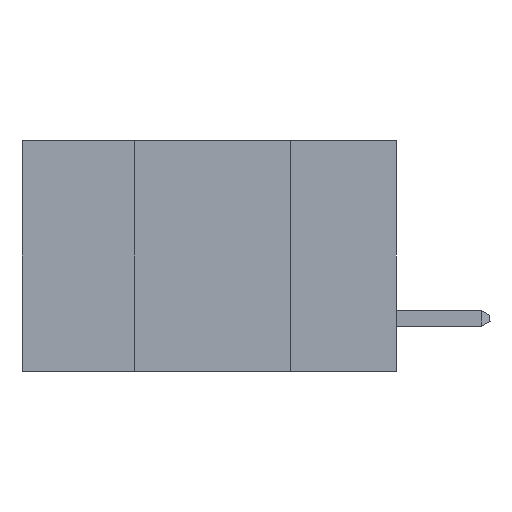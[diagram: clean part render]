
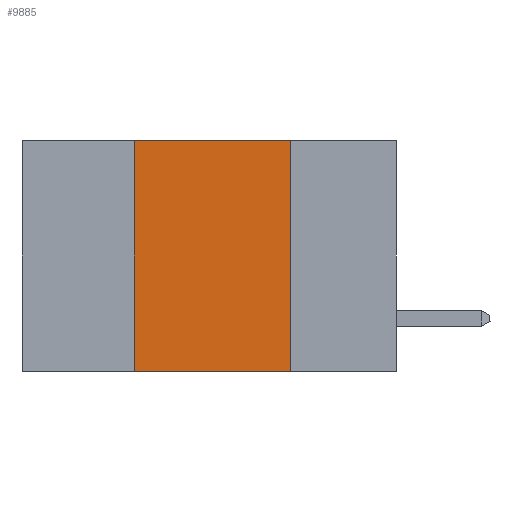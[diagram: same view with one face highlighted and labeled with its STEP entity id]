
A CAD part, left-side view. The second image highlights one B-rep face of the part: STEP entity #9885.
In plain terms, the highlighted planar face has unit normal (-1, 0, 0).
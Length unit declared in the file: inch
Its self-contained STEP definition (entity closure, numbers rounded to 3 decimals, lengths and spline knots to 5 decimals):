
#579 = DIRECTION ( 'NONE',  ( 1., 0., 0. ) ) ;
#890 = EDGE_CURVE ( 'NONE', #13135, #945, #5892, .T. ) ;
#945 = VERTEX_POINT ( 'NONE', #5460 ) ;
#1436 = FACE_OUTER_BOUND ( 'NONE', #1524, .T. ) ;
#1524 = EDGE_LOOP ( 'NONE', ( #4913, #10911, #11095, #12027 ) ) ;
#1895 = VERTEX_POINT ( 'NONE', #6417 ) ;
#2064 = CARTESIAN_POINT ( 'NONE',  ( 0., 0.6, -0.37 ) ) ;
#3016 = EDGE_CURVE ( 'NONE', #1895, #945, #7089, .T. ) ;
#3030 = VECTOR ( 'NONE', #8093, 39.37008 ) ;
#3588 = DIRECTION ( 'NONE',  ( 0., 0., -1. ) ) ;
#3705 = CARTESIAN_POINT ( 'NONE',  ( 0., 0.42, 0. ) ) ;
#4913 = ORIENTED_EDGE ( 'NONE', *, *, #890, .F. ) ;
#5460 = CARTESIAN_POINT ( 'NONE',  ( 0., 0.17, -0.37 ) ) ;
#5790 = DIRECTION ( 'NONE',  ( 0., -1., 0. ) ) ;
#5892 = LINE ( 'NONE', #10399, #9360 ) ;
#5933 = AXIS2_PLACEMENT_3D ( 'NONE', #13184, #579, #3588 ) ;
#5948 = CARTESIAN_POINT ( 'NONE',  ( 0., 0.42, 0. ) ) ;
#6417 = CARTESIAN_POINT ( 'NONE',  ( 0., 0.42, -0.37 ) ) ;
#7089 = LINE ( 'NONE', #2064, #12997 ) ;
#7203 = CARTESIAN_POINT ( 'NONE',  ( 0., 0.17, 0. ) ) ;
#7704 = CARTESIAN_POINT ( 'NONE',  ( 0., 0.6, 0. ) ) ;
#7819 = EDGE_CURVE ( 'NONE', #1895, #10705, #8576, .T. ) ;
#8093 = DIRECTION ( 'NONE',  ( 0., 0., 1. ) ) ;
#8576 = LINE ( 'NONE', #5948, #3030 ) ;
#8917 = PLANE ( 'NONE',  #5933 ) ;
#9360 = VECTOR ( 'NONE', #11675, 39.37008 ) ;
#9381 = DIRECTION ( 'NONE',  ( 0., -1., 0. ) ) ;
#9885 = ADVANCED_FACE ( 'NONE', ( #1436 ), #8917, .F. ) ;
#10399 = CARTESIAN_POINT ( 'NONE',  ( 0., 0.17, 0. ) ) ;
#10705 = VERTEX_POINT ( 'NONE', #3705 ) ;
#10911 = ORIENTED_EDGE ( 'NONE', *, *, #12844, .F. ) ;
#11095 = ORIENTED_EDGE ( 'NONE', *, *, #7819, .F. ) ;
#11250 = VECTOR ( 'NONE', #5790, 39.37008 ) ;
#11675 = DIRECTION ( 'NONE',  ( 0., 0., -1. ) ) ;
#11895 = LINE ( 'NONE', #7704, #11250 ) ;
#12027 = ORIENTED_EDGE ( 'NONE', *, *, #3016, .T. ) ;
#12844 = EDGE_CURVE ( 'NONE', #10705, #13135, #11895, .T. ) ;
#12997 = VECTOR ( 'NONE', #9381, 39.37008 ) ;
#13135 = VERTEX_POINT ( 'NONE', #7203 ) ;
#13184 = CARTESIAN_POINT ( 'NONE',  ( 0., 0.6, 0. ) ) ;
